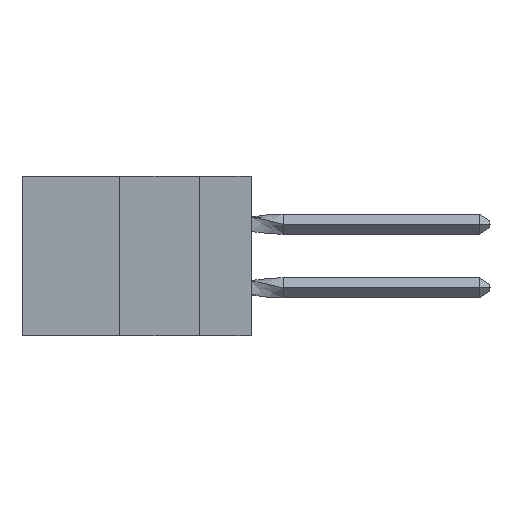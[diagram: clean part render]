
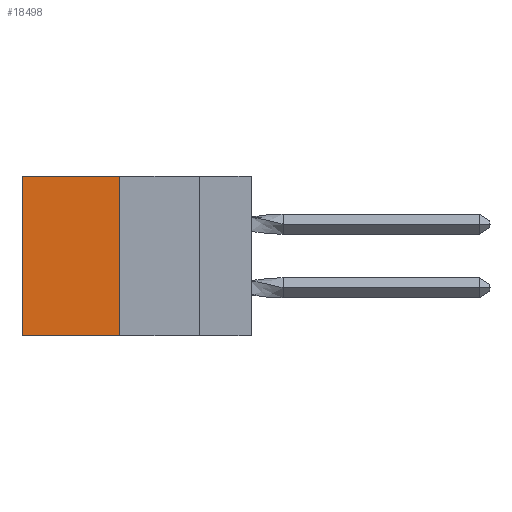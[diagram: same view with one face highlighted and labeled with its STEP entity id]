
A CAD part, left-side view. The second image highlights one B-rep face of the part: STEP entity #18498.
In plain terms, the highlighted planar face has unit normal (-1, 0, 0).
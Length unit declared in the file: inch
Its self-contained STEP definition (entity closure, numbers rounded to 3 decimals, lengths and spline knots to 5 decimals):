
#4264 = LINE ( 'NONE', #6259, #18583 ) ;
#6259 = CARTESIAN_POINT ( 'NONE',  ( 0.305, 0.413, 0. ) ) ;
#6383 = FACE_OUTER_BOUND ( 'NONE', #13350, .T. ) ;
#6430 = DIRECTION ( 'NONE',  ( 0., 0., -1. ) ) ;
#7518 = LINE ( 'NONE', #26871, #16621 ) ;
#7632 = CARTESIAN_POINT ( 'NONE',  ( 0.305, 0.413, -0.5 ) ) ;
#8102 = DIRECTION ( 'NONE',  ( 0., 1., 0. ) ) ;
#8438 = VERTEX_POINT ( 'NONE', #15713 ) ;
#9524 = DIRECTION ( 'NONE',  ( 1., 0., 0. ) ) ;
#9661 = EDGE_CURVE ( 'NONE', #8438, #25020, #19005, .T. ) ;
#9682 = AXIS2_PLACEMENT_3D ( 'NONE', #7632, #9524, #15718 ) ;
#11243 = VERTEX_POINT ( 'NONE', #19658 ) ;
#11360 = EDGE_CURVE ( 'NONE', #21203, #11243, #4264, .T. ) ;
#12149 = CARTESIAN_POINT ( 'NONE',  ( 0.305, 0.413, -0.5 ) ) ;
#12544 = ORIENTED_EDGE ( 'NONE', *, *, #19407, .F. ) ;
#12867 = CARTESIAN_POINT ( 'NONE',  ( 0.305, 0.413, 0. ) ) ;
#13350 = EDGE_LOOP ( 'NONE', ( #15894, #19100, #12544, #22600 ) ) ;
#15713 = CARTESIAN_POINT ( 'NONE',  ( 0.305, 0.413, -0.5 ) ) ;
#15718 = DIRECTION ( 'NONE',  ( 0., 0., -1. ) ) ;
#15752 = LINE ( 'NONE', #21204, #21917 ) ;
#15894 = ORIENTED_EDGE ( 'NONE', *, *, #25934, .T. ) ;
#16621 = VECTOR ( 'NONE', #24395, 39.37008 ) ;
#18200 = DIRECTION ( 'NONE',  ( 0., 1., 0. ) ) ;
#18498 = ADVANCED_FACE ( 'NONE', ( #6383 ), #21973, .F. ) ;
#18583 = VECTOR ( 'NONE', #8102, 39.37008 ) ;
#19005 = LINE ( 'NONE', #12149, #20949 ) ;
#19100 = ORIENTED_EDGE ( 'NONE', *, *, #9661, .F. ) ;
#19407 = EDGE_CURVE ( 'NONE', #21203, #8438, #15752, .T. ) ;
#19658 = CARTESIAN_POINT ( 'NONE',  ( 0.305, 0.72, 0. ) ) ;
#20949 = VECTOR ( 'NONE', #18200, 39.37008 ) ;
#21203 = VERTEX_POINT ( 'NONE', #12867 ) ;
#21204 = CARTESIAN_POINT ( 'NONE',  ( 0.305, 0.413, -0.5 ) ) ;
#21917 = VECTOR ( 'NONE', #6430, 39.37008 ) ;
#21973 = PLANE ( 'NONE',  #9682 ) ;
#22600 = ORIENTED_EDGE ( 'NONE', *, *, #11360, .T. ) ;
#23245 = CARTESIAN_POINT ( 'NONE',  ( 0.305, 0.72, -0.5 ) ) ;
#24395 = DIRECTION ( 'NONE',  ( 0., 0., -1. ) ) ;
#25020 = VERTEX_POINT ( 'NONE', #23245 ) ;
#25934 = EDGE_CURVE ( 'NONE', #11243, #25020, #7518, .T. ) ;
#26871 = CARTESIAN_POINT ( 'NONE',  ( 0.305, 0.72, -0.5 ) ) ;
